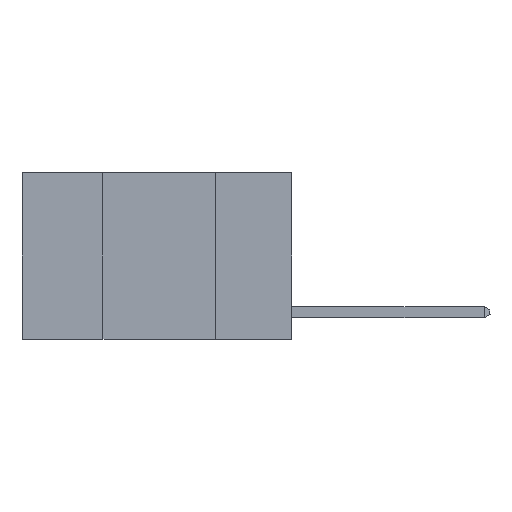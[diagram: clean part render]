
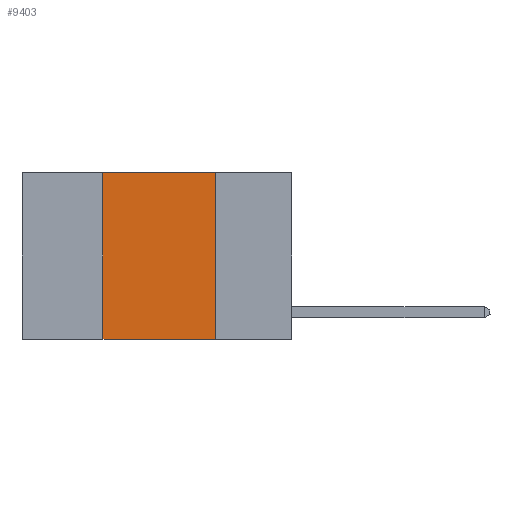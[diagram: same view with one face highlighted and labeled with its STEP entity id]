
A CAD part, left-side view. The second image highlights one B-rep face of the part: STEP entity #9403.
In plain terms, the highlighted planar face has unit normal (-1, 0, 0).
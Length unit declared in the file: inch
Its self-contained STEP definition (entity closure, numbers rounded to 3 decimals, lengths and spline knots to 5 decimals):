
#131 = DIRECTION ( 'NONE',  ( 0., -1., 0. ) ) ;
#758 = CARTESIAN_POINT ( 'NONE',  ( 0., 0.17, -0.37 ) ) ;
#912 = DIRECTION ( 'NONE',  ( 0., 0., 1. ) ) ;
#1914 = CARTESIAN_POINT ( 'NONE',  ( 0., 0.6, -0.37 ) ) ;
#2561 = CARTESIAN_POINT ( 'NONE',  ( 0., 0.6, 0. ) ) ;
#4229 = LINE ( 'NONE', #2561, #13217 ) ;
#5765 = DIRECTION ( 'NONE',  ( 0., 0., -1. ) ) ;
#5900 = CARTESIAN_POINT ( 'NONE',  ( 0., 0.6, 0. ) ) ;
#6054 = VERTEX_POINT ( 'NONE', #758 ) ;
#6941 = DIRECTION ( 'NONE',  ( 0., 0., -1. ) ) ;
#8006 = DIRECTION ( 'NONE',  ( 1., 0., 0. ) ) ;
#9314 = LINE ( 'NONE', #25944, #26057 ) ;
#9403 = ADVANCED_FACE ( 'NONE', ( #25046 ), #22421, .F. ) ;
#9961 = VECTOR ( 'NONE', #131, 39.37008 ) ;
#11467 = LINE ( 'NONE', #18253, #17265 ) ;
#12506 = CARTESIAN_POINT ( 'NONE',  ( 0., 0.42, 0. ) ) ;
#12985 = ORIENTED_EDGE ( 'NONE', *, *, #24553, .F. ) ;
#13217 = VECTOR ( 'NONE', #23257, 39.37008 ) ;
#13598 = AXIS2_PLACEMENT_3D ( 'NONE', #5900, #8006, #5765 ) ;
#13618 = ORIENTED_EDGE ( 'NONE', *, *, #26827, .F. ) ;
#13752 = CARTESIAN_POINT ( 'NONE',  ( 0., 0.17, 0. ) ) ;
#14095 = EDGE_CURVE ( 'NONE', #25200, #21800, #11467, .T. ) ;
#15285 = ORIENTED_EDGE ( 'NONE', *, *, #14095, .F. ) ;
#17265 = VECTOR ( 'NONE', #912, 39.37008 ) ;
#17657 = CARTESIAN_POINT ( 'NONE',  ( 0., 0.42, -0.37 ) ) ;
#18253 = CARTESIAN_POINT ( 'NONE',  ( 0., 0.42, 0. ) ) ;
#20660 = EDGE_CURVE ( 'NONE', #25200, #6054, #23156, .T. ) ;
#21800 = VERTEX_POINT ( 'NONE', #12506 ) ;
#22421 = PLANE ( 'NONE',  #13598 ) ;
#23156 = LINE ( 'NONE', #1914, #9961 ) ;
#23257 = DIRECTION ( 'NONE',  ( 0., -1., 0. ) ) ;
#24553 = EDGE_CURVE ( 'NONE', #21800, #26820, #4229, .T. ) ;
#25046 = FACE_OUTER_BOUND ( 'NONE', #27129, .T. ) ;
#25200 = VERTEX_POINT ( 'NONE', #17657 ) ;
#25944 = CARTESIAN_POINT ( 'NONE',  ( 0., 0.17, 0. ) ) ;
#26057 = VECTOR ( 'NONE', #6941, 39.37008 ) ;
#26820 = VERTEX_POINT ( 'NONE', #13752 ) ;
#26827 = EDGE_CURVE ( 'NONE', #26820, #6054, #9314, .T. ) ;
#27096 = ORIENTED_EDGE ( 'NONE', *, *, #20660, .T. ) ;
#27129 = EDGE_LOOP ( 'NONE', ( #13618, #12985, #15285, #27096 ) ) ;
